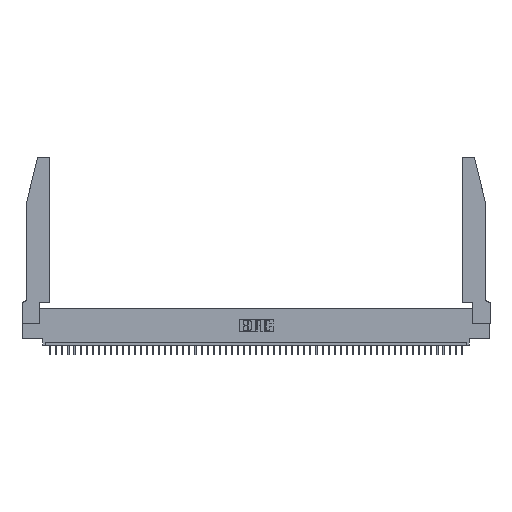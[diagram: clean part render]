
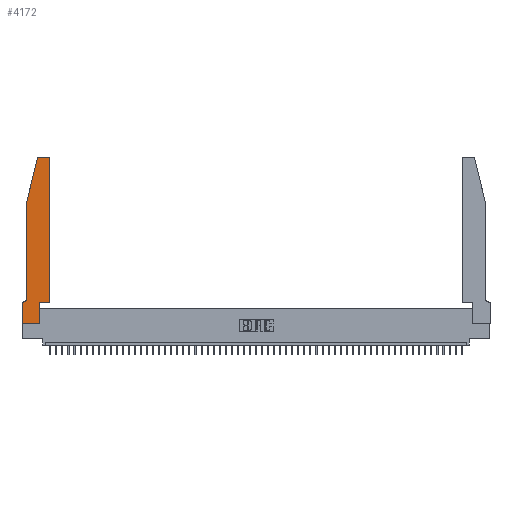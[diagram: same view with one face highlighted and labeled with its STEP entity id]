
A CAD part, top view. The second image highlights one B-rep face of the part: STEP entity #4172.
In plain terms, the highlighted planar face has unit normal (0, 0, 1).
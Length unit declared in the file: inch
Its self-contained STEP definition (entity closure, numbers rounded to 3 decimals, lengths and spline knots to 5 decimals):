
#276 = LINE ( 'NONE', #51438, #30495 ) ;
#1360 = EDGE_CURVE ( 'NONE', #31200, #22417, #34416, .T. ) ;
#3529 = PLANE ( 'NONE',  #30274 ) ;
#3939 = ORIENTED_EDGE ( 'NONE', *, *, #1360, .T. ) ;
#4172 = ADVANCED_FACE ( 'NONE', ( #10923 ), #3529, .T. ) ;
#4263 = CARTESIAN_POINT ( 'NONE',  ( 0.4505, 0.35, 0.37 ) ) ;
#4502 = CARTESIAN_POINT ( 'NONE',  ( 0.0755, 2., 0.37 ) ) ;
#5145 = AXIS2_PLACEMENT_3D ( 'NONE', #36321, #7928, #24846 ) ;
#5960 = EDGE_CURVE ( 'NONE', #49582, #16608, #19247, .T. ) ;
#6079 = ORIENTED_EDGE ( 'NONE', *, *, #21568, .T. ) ;
#6348 = VECTOR ( 'NONE', #21301, 39.37008 ) ;
#7928 = DIRECTION ( 'NONE',  ( 0., 0., -1. ) ) ;
#8507 = DIRECTION ( 'NONE',  ( 0., -1., 0. ) ) ;
#8871 = CARTESIAN_POINT ( 'NONE',  ( 0.4505, 0.35, 0.37 ) ) ;
#9193 = ORIENTED_EDGE ( 'NONE', *, *, #18978, .T. ) ;
#10173 = LINE ( 'NONE', #46069, #43618 ) ;
#10403 = AXIS2_PLACEMENT_3D ( 'NONE', #49896, #33386, #12561 ) ;
#10923 = FACE_OUTER_BOUND ( 'NONE', #20988, .T. ) ;
#11032 = DIRECTION ( 'NONE',  ( 0., 0., 1. ) ) ;
#11310 = LINE ( 'NONE', #13260, #49869 ) ;
#11515 = LINE ( 'NONE', #12153, #24356 ) ;
#12153 = CARTESIAN_POINT ( 'NONE',  ( 0., 0., 0.37 ) ) ;
#12336 = CARTESIAN_POINT ( 'NONE',  ( 0.0755, 2., 0.37 ) ) ;
#12561 = DIRECTION ( 'NONE',  ( 1., 0., 0. ) ) ;
#13260 = CARTESIAN_POINT ( 'NONE',  ( 0.0755, 2., 0.37 ) ) ;
#13854 = CARTESIAN_POINT ( 'NONE',  ( 0.0055, 0.35, 0.37 ) ) ;
#14083 = DIRECTION ( 'NONE',  ( -1., 0., 0. ) ) ;
#14470 = CARTESIAN_POINT ( 'NONE',  ( 0.4205, 2.72, 0.37 ) ) ;
#14514 = EDGE_CURVE ( 'NONE', #42648, #20480, #276, .T. ) ;
#15165 = ORIENTED_EDGE ( 'NONE', *, *, #39751, .T. ) ;
#16114 = EDGE_CURVE ( 'NONE', #32793, #31200, #49637, .T. ) ;
#16608 = VERTEX_POINT ( 'NONE', #52360 ) ;
#18102 = CARTESIAN_POINT ( 'NONE',  ( 0.2865, 0., 0.37 ) ) ;
#18940 = ORIENTED_EDGE ( 'NONE', *, *, #16114, .T. ) ;
#18978 = EDGE_CURVE ( 'NONE', #44134, #32793, #51211, .T. ) ;
#19006 = EDGE_CURVE ( 'NONE', #24908, #49582, #11515, .T. ) ;
#19247 = LINE ( 'NONE', #33546, #6348 ) ;
#19616 = CARTESIAN_POINT ( 'NONE',  ( 0.0755, 0.42, 0.37 ) ) ;
#20480 = VERTEX_POINT ( 'NONE', #25816 ) ;
#20988 = EDGE_LOOP ( 'NONE', ( #40228, #6079, #35942, #9193, #18940, #3939, #15165, #27922, #33061, #32453, #32480, #44084 ) ) ;
#21028 = LINE ( 'NONE', #34620, #52537 ) ;
#21301 = DIRECTION ( 'NONE',  ( 0., 1., 0. ) ) ;
#21414 = CARTESIAN_POINT ( 'NONE',  ( 0.4205, 2.75, 0.37 ) ) ;
#21568 = EDGE_CURVE ( 'NONE', #20480, #38124, #27964, .T. ) ;
#22417 = VERTEX_POINT ( 'NONE', #48856 ) ;
#22934 = EDGE_CURVE ( 'NONE', #48123, #49255, #45828, .T. ) ;
#23523 = VECTOR ( 'NONE', #26882, 39.37008 ) ;
#24170 = CIRCLE ( 'NONE', #47168, 0.03 ) ;
#24253 = CARTESIAN_POINT ( 'NONE',  ( 0., 0., 0.37 ) ) ;
#24356 = VECTOR ( 'NONE', #48974, 39.37008 ) ;
#24846 = DIRECTION ( 'NONE',  ( -1., 0., 0. ) ) ;
#24908 = VERTEX_POINT ( 'NONE', #24253 ) ;
#25568 = DIRECTION ( 'NONE',  ( 0., -1., 0. ) ) ;
#25816 = CARTESIAN_POINT ( 'NONE',  ( 0.284, 2.75, 0.37 ) ) ;
#26882 = DIRECTION ( 'NONE',  ( -1., 0., 0. ) ) ;
#27922 = ORIENTED_EDGE ( 'NONE', *, *, #19006, .T. ) ;
#27964 = CIRCLE ( 'NONE', #10403, 0.03 ) ;
#30274 = AXIS2_PLACEMENT_3D ( 'NONE', #49022, #44897, #48832 ) ;
#30495 = VECTOR ( 'NONE', #14083, 39.37008 ) ;
#31200 = VERTEX_POINT ( 'NONE', #13854 ) ;
#31750 = EDGE_CURVE ( 'NONE', #16608, #48123, #21028, .T. ) ;
#32453 = ORIENTED_EDGE ( 'NONE', *, *, #31750, .T. ) ;
#32480 = ORIENTED_EDGE ( 'NONE', *, *, #22934, .T. ) ;
#32793 = VERTEX_POINT ( 'NONE', #19616 ) ;
#33061 = ORIENTED_EDGE ( 'NONE', *, *, #5960, .T. ) ;
#33386 = DIRECTION ( 'NONE',  ( 0., 0., 1. ) ) ;
#33546 = CARTESIAN_POINT ( 'NONE',  ( 0.2865, 0.35, 0.37 ) ) ;
#34203 = VECTOR ( 'NONE', #36817, 39.37008 ) ;
#34416 = LINE ( 'NONE', #51527, #23523 ) ;
#34620 = CARTESIAN_POINT ( 'NONE',  ( 0.4505, 0.35, 0.37 ) ) ;
#34986 = DIRECTION ( 'NONE',  ( 1., 0., 0. ) ) ;
#35942 = ORIENTED_EDGE ( 'NONE', *, *, #52177, .T. ) ;
#36321 = CARTESIAN_POINT ( 'NONE',  ( 0.0055, 0.42, 0.37 ) ) ;
#36817 = DIRECTION ( 'NONE',  ( 0., 1., 0. ) ) ;
#38124 = VERTEX_POINT ( 'NONE', #51251 ) ;
#39437 = DIRECTION ( 'NONE',  ( 1., 0., 0. ) ) ;
#39751 = EDGE_CURVE ( 'NONE', #22417, #24908, #10173, .T. ) ;
#40228 = ORIENTED_EDGE ( 'NONE', *, *, #14514, .T. ) ;
#42255 = EDGE_CURVE ( 'NONE', #49255, #42648, #24170, .T. ) ;
#42648 = VERTEX_POINT ( 'NONE', #21414 ) ;
#43618 = VECTOR ( 'NONE', #25568, 39.37008 ) ;
#44084 = ORIENTED_EDGE ( 'NONE', *, *, #42255, .T. ) ;
#44134 = VERTEX_POINT ( 'NONE', #4502 ) ;
#44897 = DIRECTION ( 'NONE',  ( 0., 0., 1. ) ) ;
#45828 = LINE ( 'NONE', #4263, #34203 ) ;
#46069 = CARTESIAN_POINT ( 'NONE',  ( 0., 0., 0.37 ) ) ;
#47168 = AXIS2_PLACEMENT_3D ( 'NONE', #14470, #11032, #39437 ) ;
#47681 = VECTOR ( 'NONE', #8507, 39.37008 ) ;
#48123 = VERTEX_POINT ( 'NONE', #8871 ) ;
#48832 = DIRECTION ( 'NONE',  ( 1., 0., 0. ) ) ;
#48856 = CARTESIAN_POINT ( 'NONE',  ( 0., 0.35, 0.37 ) ) ;
#48974 = DIRECTION ( 'NONE',  ( 1., 0., 0. ) ) ;
#49022 = CARTESIAN_POINT ( 'NONE',  ( 0., 0.35, 0.37 ) ) ;
#49255 = VERTEX_POINT ( 'NONE', #52109 ) ;
#49582 = VERTEX_POINT ( 'NONE', #18102 ) ;
#49637 = CIRCLE ( 'NONE', #5145, 0.07 ) ;
#49726 = DIRECTION ( 'NONE',  ( -0.239, -0.971, 0. ) ) ;
#49869 = VECTOR ( 'NONE', #49726, 39.37008 ) ;
#49896 = CARTESIAN_POINT ( 'NONE',  ( 0.284, 2.72, 0.37 ) ) ;
#51211 = LINE ( 'NONE', #12336, #47681 ) ;
#51251 = CARTESIAN_POINT ( 'NONE',  ( 0.25487, 2.72718, 0.37 ) ) ;
#51438 = CARTESIAN_POINT ( 'NONE',  ( 0.2605, 2.75, 0.37 ) ) ;
#51527 = CARTESIAN_POINT ( 'NONE',  ( 0.0755, 0.35, 0.37 ) ) ;
#52109 = CARTESIAN_POINT ( 'NONE',  ( 0.4505, 2.72, 0.37 ) ) ;
#52177 = EDGE_CURVE ( 'NONE', #38124, #44134, #11310, .T. ) ;
#52360 = CARTESIAN_POINT ( 'NONE',  ( 0.2865, 0.35, 0.37 ) ) ;
#52537 = VECTOR ( 'NONE', #34986, 39.37008 ) ;
